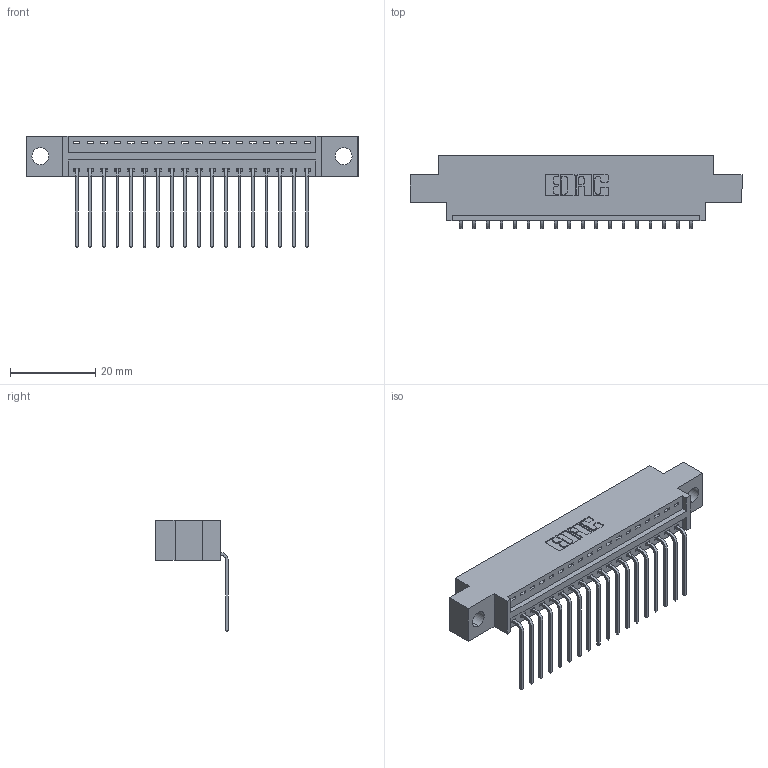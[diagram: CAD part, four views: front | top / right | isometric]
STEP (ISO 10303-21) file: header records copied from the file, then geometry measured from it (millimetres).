
FILE_DESCRIPTION (( 'STEP AP203' ), '1' );
FILE_NAME ('346-018-559-604.STEP', '2022-05-05T14:44:07', ( '' ), ( '' ), 'SwSTEP 2.0', 'SolidWorks 2020', '' );
FILE_SCHEMA (( 'CONFIG_CONTROL_DESIGN' ));
Length unit declared in the file: inch
Products named in the file (3): 345-292-001_558 559 Tail - 1; 346-018-559-604; 346 Part_0.170 Offset - 0.156 Dia-TH
Assembly tree (19 placements, depth 2):
  346-018-559-604
    346 Part_0.170 Offset - 0.156 Dia-TH
    345-292-001_558 559 Tail - 1  x18
Bounding box: 77.72 x 17.08 x 26.16 mm (x, y, z)
Volume: 7074 mm3; surface area: 8937.9 mm2
Topology: 19 solids, 19 shells, 1220 faces, 3653 edges, 2410 vertices
Faces by surface type: plane 850, cylinder 370
Entity records: 15037 total; most frequent: CARTESIAN_POINT 2596, ORIENTED_EDGE 2546, DIRECTION 2317, EDGE_CURVE 1273, VECTOR 1069, LINE 1069, VERTEX_POINT 846, AXIS2_PLACEMENT_3D 624
